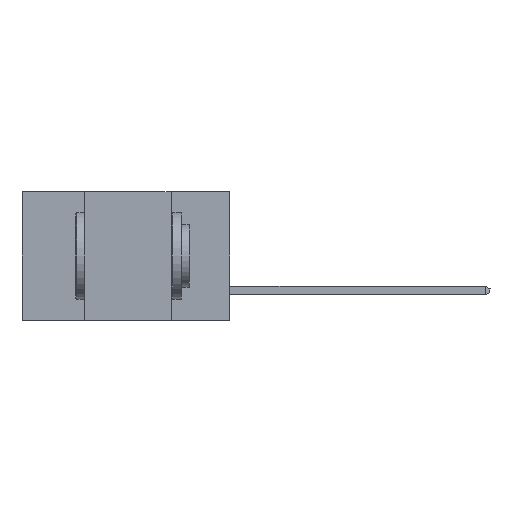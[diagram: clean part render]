
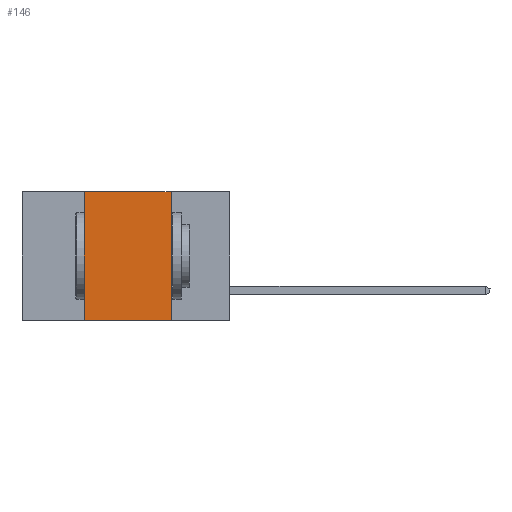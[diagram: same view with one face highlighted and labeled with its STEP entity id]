
A CAD part, left-side view. The second image highlights one B-rep face of the part: STEP entity #146.
In plain terms, the highlighted planar face has unit normal (-1, 0, 0).
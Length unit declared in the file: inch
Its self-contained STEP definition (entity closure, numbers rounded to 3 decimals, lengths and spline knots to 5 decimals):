
#146 = ADVANCED_FACE ( 'NONE', ( #6878 ), #2540, .F. ) ;
#354 = VECTOR ( 'NONE', #9727, 39.37008 ) ;
#1376 = EDGE_CURVE ( 'NONE', #7456, #5179, #7696, .T. ) ;
#2017 = CARTESIAN_POINT ( 'NONE',  ( 0., 0.17, 0. ) ) ;
#2135 = VECTOR ( 'NONE', #9650, 39.37008 ) ;
#2540 = PLANE ( 'NONE',  #8143 ) ;
#2676 = DIRECTION ( 'NONE',  ( 0., -1., 0. ) ) ;
#2768 = ORIENTED_EDGE ( 'NONE', *, *, #3212, .F. ) ;
#2831 = DIRECTION ( 'NONE',  ( 0., 0., -1. ) ) ;
#2934 = EDGE_CURVE ( 'NONE', #9089, #6352, #8085, .T. ) ;
#3170 = ORIENTED_EDGE ( 'NONE', *, *, #2934, .F. ) ;
#3212 = EDGE_CURVE ( 'NONE', #6352, #5179, #6188, .T. ) ;
#3779 = CARTESIAN_POINT ( 'NONE',  ( 0., 0.17, -0.37 ) ) ;
#4555 = VECTOR ( 'NONE', #2831, 39.37008 ) ;
#5179 = VERTEX_POINT ( 'NONE', #8462 ) ;
#5821 = CARTESIAN_POINT ( 'NONE',  ( 0., 0.6, -0.37 ) ) ;
#5943 = DIRECTION ( 'NONE',  ( 0., 0., -1. ) ) ;
#6188 = LINE ( 'NONE', #3779, #4555 ) ;
#6352 = VERTEX_POINT ( 'NONE', #2017 ) ;
#6797 = EDGE_CURVE ( 'NONE', #7456, #9089, #8179, .T. ) ;
#6878 = FACE_OUTER_BOUND ( 'NONE', #7670, .T. ) ;
#7456 = VERTEX_POINT ( 'NONE', #8164 ) ;
#7670 = EDGE_LOOP ( 'NONE', ( #2768, #3170, #8253, #8579 ) ) ;
#7696 = LINE ( 'NONE', #5821, #10483 ) ;
#8085 = LINE ( 'NONE', #8922, #354 ) ;
#8143 = AXIS2_PLACEMENT_3D ( 'NONE', #10133, #10246, #5943 ) ;
#8164 = CARTESIAN_POINT ( 'NONE',  ( 0., 0.42, -0.37 ) ) ;
#8179 = LINE ( 'NONE', #10596, #2135 ) ;
#8253 = ORIENTED_EDGE ( 'NONE', *, *, #6797, .F. ) ;
#8462 = CARTESIAN_POINT ( 'NONE',  ( 0., 0.17, -0.37 ) ) ;
#8579 = ORIENTED_EDGE ( 'NONE', *, *, #1376, .T. ) ;
#8922 = CARTESIAN_POINT ( 'NONE',  ( 0., 0.6, 0. ) ) ;
#9089 = VERTEX_POINT ( 'NONE', #9252 ) ;
#9252 = CARTESIAN_POINT ( 'NONE',  ( 0., 0.42, 0. ) ) ;
#9650 = DIRECTION ( 'NONE',  ( 0., 0., 1. ) ) ;
#9727 = DIRECTION ( 'NONE',  ( 0., -1., 0. ) ) ;
#10133 = CARTESIAN_POINT ( 'NONE',  ( 0., 0.6, 0. ) ) ;
#10246 = DIRECTION ( 'NONE',  ( 1., 0., 0. ) ) ;
#10483 = VECTOR ( 'NONE', #2676, 39.37008 ) ;
#10596 = CARTESIAN_POINT ( 'NONE',  ( 0., 0.42, -0.37 ) ) ;
